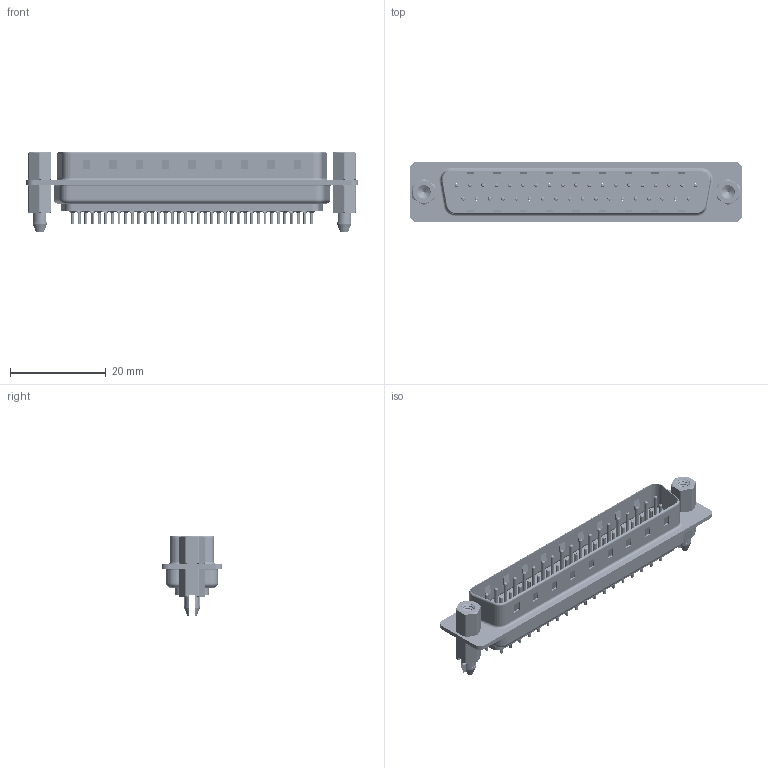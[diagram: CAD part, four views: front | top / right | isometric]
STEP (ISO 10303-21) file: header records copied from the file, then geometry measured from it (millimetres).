
FILE_DESCRIPTION (( 'STEP AP203' ), '1' );
FILE_NAME ('627-037-320-547.STEP', '2018-10-05T20:55:22', ( '' ), ( '' ), 'SwSTEP 2.0', 'SolidWorks 2016', '' );
FILE_SCHEMA (( 'CONFIG_CONTROL_DESIGN' ));
Length unit declared in the file: millimetre
Products named in the file (8): 627 4-40 Hex Standoff; 627 4-40 Threaded Boardlock_LP; 627-037-320-547; 627 Housing_37 LP; 627 Shell Front_37 Contacts; 627 Shell Rear_37 Contacts; 627 Contact Row 1_20L; 627 Contact Row 2_20L
Assembly tree (44 placements, depth 2):
  627-037-320-547
    627 Housing_37 LP
    627 Shell Front_37 Contacts
    627 Shell Rear_37 Contacts
    627 Contact Row 1_20L  x19
    627 Contact Row 2_20L  x18
    627 4-40 Hex Standoff  x2
    627 4-40 Threaded Boardlock_LP  x2
Bounding box: 69.3 x 12.6 x 16.9 mm (x, y, z)
Volume: 4009.1 mm3; surface area: 11231.2 mm2
Topology: 44 solids, 44 shells, 4238 faces, 11148 edges, 6933 vertices
Faces by surface type: cylinder 1614, plane 1145, torus 1055, cone 406, bspline 18
Entity records: 35343 total; most frequent: CARTESIAN_POINT 9856, DIRECTION 5181, ORIENTED_EDGE 4802, EDGE_CURVE 2401, AXIS2_PLACEMENT_3D 2033, VERTEX_POINT 1544, EDGE_LOOP 1163, VECTOR 1115
